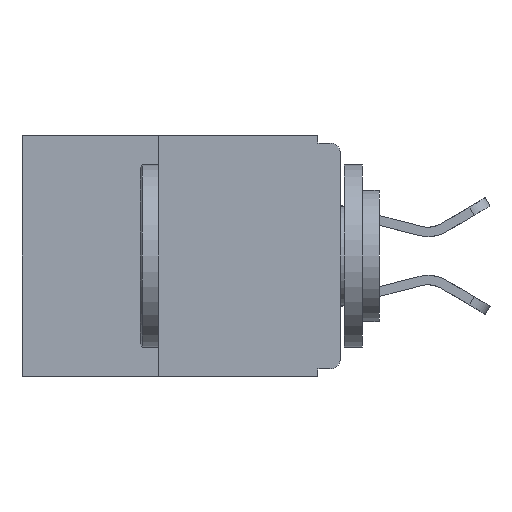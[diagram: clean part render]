
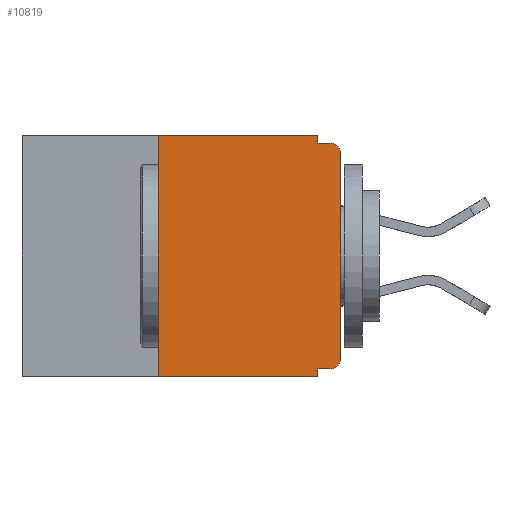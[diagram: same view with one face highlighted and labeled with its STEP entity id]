
A CAD part, left-side view. The second image highlights one B-rep face of the part: STEP entity #10819.
In plain terms, the highlighted planar face has unit normal (-1, 0, 0).
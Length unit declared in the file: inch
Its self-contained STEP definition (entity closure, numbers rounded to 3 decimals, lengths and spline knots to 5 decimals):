
#263 = VERTEX_POINT ( 'NONE', #2796 ) ;
#349 = DIRECTION ( 'NONE',  ( 0., 0., -1. ) ) ;
#385 = ORIENTED_EDGE ( 'NONE', *, *, #10585, .F. ) ;
#596 = CARTESIAN_POINT ( 'NONE',  ( 0., 0.015, -0.01 ) ) ;
#684 = EDGE_CURVE ( 'NONE', #263, #14682, #11679, .T. ) ;
#901 = EDGE_LOOP ( 'NONE', ( #12877, #3703, #15467, #6103, #385, #5699, #3279, #2535, #3131, #10748 ) ) ;
#1222 = CARTESIAN_POINT ( 'NONE',  ( 0., 0.437, 0. ) ) ;
#1249 = EDGE_CURVE ( 'NONE', #1564, #7781, #10549, .T. ) ;
#1455 = VECTOR ( 'NONE', #14753, 39.37008 ) ;
#1459 = CARTESIAN_POINT ( 'NONE',  ( 0., 0.031, 0. ) ) ;
#1564 = VERTEX_POINT ( 'NONE', #2664 ) ;
#1834 = DIRECTION ( 'NONE',  ( -1., 0., 0. ) ) ;
#1847 = VECTOR ( 'NONE', #11949, 39.37008 ) ;
#1985 = CARTESIAN_POINT ( 'NONE',  ( 0., 0.031, -0.01 ) ) ;
#2091 = VECTOR ( 'NONE', #3565, 39.37008 ) ;
#2436 = VERTEX_POINT ( 'NONE', #9599 ) ;
#2535 = ORIENTED_EDGE ( 'NONE', *, *, #6618, .F. ) ;
#2664 = CARTESIAN_POINT ( 'NONE',  ( 0., 0., -0.305 ) ) ;
#2796 = CARTESIAN_POINT ( 'NONE',  ( 0., 0.031, 0. ) ) ;
#2798 = CARTESIAN_POINT ( 'NONE',  ( 0., 0.015, -0.32 ) ) ;
#2909 = CARTESIAN_POINT ( 'NONE',  ( 0., 0.25, -0.33 ) ) ;
#2918 = LINE ( 'NONE', #1222, #9347 ) ;
#3131 = ORIENTED_EDGE ( 'NONE', *, *, #13862, .F. ) ;
#3216 = EDGE_CURVE ( 'NONE', #9391, #7124, #5348, .T. ) ;
#3255 = VERTEX_POINT ( 'NONE', #2798 ) ;
#3279 = ORIENTED_EDGE ( 'NONE', *, *, #3216, .T. ) ;
#3506 = DIRECTION ( 'NONE',  ( -1., 0., 0. ) ) ;
#3565 = DIRECTION ( 'NONE',  ( 0., -1., 0. ) ) ;
#3703 = ORIENTED_EDGE ( 'NONE', *, *, #15349, .T. ) ;
#4077 = DIRECTION ( 'NONE',  ( 0., 0., -1. ) ) ;
#4089 = PLANE ( 'NONE',  #13505 ) ;
#4157 = DIRECTION ( 'NONE',  ( 0., 0., 1. ) ) ;
#4318 = VECTOR ( 'NONE', #11403, 39.37008 ) ;
#4879 = AXIS2_PLACEMENT_3D ( 'NONE', #9106, #1834, #10356 ) ;
#5290 = CARTESIAN_POINT ( 'NONE',  ( 0., 0.437, 0. ) ) ;
#5348 = LINE ( 'NONE', #13688, #2091 ) ;
#5482 = VERTEX_POINT ( 'NONE', #12395 ) ;
#5581 = CARTESIAN_POINT ( 'NONE',  ( 0., 0.031, -0.33 ) ) ;
#5699 = ORIENTED_EDGE ( 'NONE', *, *, #7592, .F. ) ;
#6103 = ORIENTED_EDGE ( 'NONE', *, *, #684, .F. ) ;
#6618 = EDGE_CURVE ( 'NONE', #5482, #7124, #8682, .T. ) ;
#7124 = VERTEX_POINT ( 'NONE', #5581 ) ;
#7318 = VECTOR ( 'NONE', #4157, 39.37008 ) ;
#7556 = CARTESIAN_POINT ( 'NONE',  ( 0., 0., -0.32 ) ) ;
#7592 = EDGE_CURVE ( 'NONE', #9391, #2436, #13188, .T. ) ;
#7718 = DIRECTION ( 'NONE',  ( 1., 0., 0. ) ) ;
#7781 = VERTEX_POINT ( 'NONE', #15328 ) ;
#8039 = LINE ( 'NONE', #11923, #14062 ) ;
#8414 = CIRCLE ( 'NONE', #4879, 0.015 ) ;
#8444 = VECTOR ( 'NONE', #4077, 39.37008 ) ;
#8682 = LINE ( 'NONE', #10762, #1847 ) ;
#9106 = CARTESIAN_POINT ( 'NONE',  ( 0., 0.015, -0.305 ) ) ;
#9347 = VECTOR ( 'NONE', #9750, 39.37008 ) ;
#9391 = VERTEX_POINT ( 'NONE', #15628 ) ;
#9599 = CARTESIAN_POINT ( 'NONE',  ( 0., 0.25, 0. ) ) ;
#9750 = DIRECTION ( 'NONE',  ( 0., -1., 0. ) ) ;
#10356 = DIRECTION ( 'NONE',  ( 0., 0., -1. ) ) ;
#10396 = VERTEX_POINT ( 'NONE', #596 ) ;
#10461 = EDGE_CURVE ( 'NONE', #14682, #10396, #8039, .T. ) ;
#10549 = LINE ( 'NONE', #12712, #7318 ) ;
#10585 = EDGE_CURVE ( 'NONE', #2436, #263, #2918, .T. ) ;
#10748 = ORIENTED_EDGE ( 'NONE', *, *, #12780, .T. ) ;
#10762 = CARTESIAN_POINT ( 'NONE',  ( 0., 0.031, -0.33 ) ) ;
#10794 = LINE ( 'NONE', #7556, #1455 ) ;
#10804 = CARTESIAN_POINT ( 'NONE',  ( 0., 0.015, -0.025 ) ) ;
#10819 = ADVANCED_FACE ( 'NONE', ( #12369 ), #4089, .F. ) ;
#11403 = DIRECTION ( 'NONE',  ( 0., 0., 1. ) ) ;
#11679 = LINE ( 'NONE', #1459, #8444 ) ;
#11923 = CARTESIAN_POINT ( 'NONE',  ( 0., 0., -0.01 ) ) ;
#11949 = DIRECTION ( 'NONE',  ( 0., 0., -1. ) ) ;
#11990 = DIRECTION ( 'NONE',  ( 0., 0., -1. ) ) ;
#12369 = FACE_OUTER_BOUND ( 'NONE', #901, .T. ) ;
#12395 = CARTESIAN_POINT ( 'NONE',  ( 0., 0.031, -0.32 ) ) ;
#12712 = CARTESIAN_POINT ( 'NONE',  ( 0., 0., 0. ) ) ;
#12780 = EDGE_CURVE ( 'NONE', #3255, #1564, #8414, .T. ) ;
#12877 = ORIENTED_EDGE ( 'NONE', *, *, #1249, .T. ) ;
#13111 = DIRECTION ( 'NONE',  ( 0., -1., 0. ) ) ;
#13188 = LINE ( 'NONE', #2909, #4318 ) ;
#13505 = AXIS2_PLACEMENT_3D ( 'NONE', #5290, #7718, #349 ) ;
#13688 = CARTESIAN_POINT ( 'NONE',  ( 0., 0.437, -0.33 ) ) ;
#13862 = EDGE_CURVE ( 'NONE', #3255, #5482, #10794, .T. ) ;
#14062 = VECTOR ( 'NONE', #13111, 39.37008 ) ;
#14470 = CIRCLE ( 'NONE', #15117, 0.015 ) ;
#14682 = VERTEX_POINT ( 'NONE', #1985 ) ;
#14753 = DIRECTION ( 'NONE',  ( 0., 1., 0. ) ) ;
#15117 = AXIS2_PLACEMENT_3D ( 'NONE', #10804, #3506, #11990 ) ;
#15328 = CARTESIAN_POINT ( 'NONE',  ( 0., 0., -0.025 ) ) ;
#15349 = EDGE_CURVE ( 'NONE', #7781, #10396, #14470, .T. ) ;
#15467 = ORIENTED_EDGE ( 'NONE', *, *, #10461, .F. ) ;
#15628 = CARTESIAN_POINT ( 'NONE',  ( 0., 0.25, -0.33 ) ) ;
